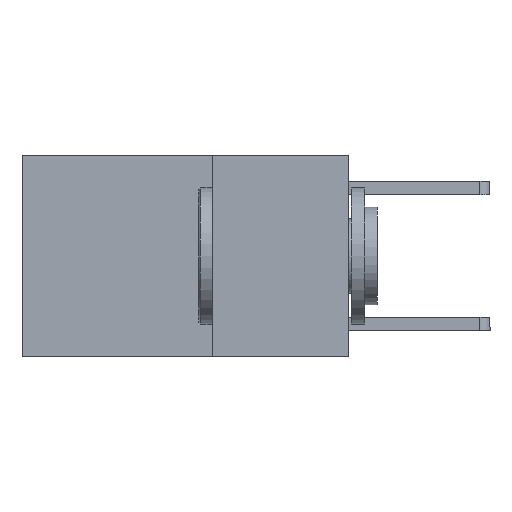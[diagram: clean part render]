
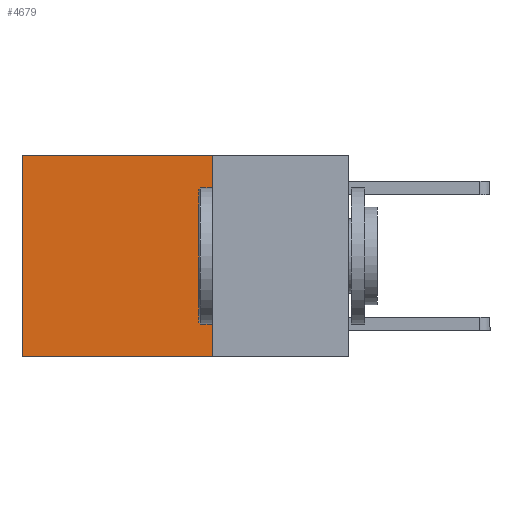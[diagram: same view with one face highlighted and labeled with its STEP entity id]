
A CAD part, left-side view. The second image highlights one B-rep face of the part: STEP entity #4679.
In plain terms, the highlighted planar face has unit normal (-1, 0, 0).
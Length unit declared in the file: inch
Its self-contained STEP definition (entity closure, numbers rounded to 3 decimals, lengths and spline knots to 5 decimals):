
#667 = LINE ( 'NONE', #8625, #9826 ) ;
#1296 = VECTOR ( 'NONE', #3431, 39.37008 ) ;
#1377 = VECTOR ( 'NONE', #4967, 39.37008 ) ;
#1406 = PLANE ( 'NONE',  #5286 ) ;
#1870 = VERTEX_POINT ( 'NONE', #2147 ) ;
#2147 = CARTESIAN_POINT ( 'NONE',  ( 0.2625, 0.25, 0. ) ) ;
#2241 = VERTEX_POINT ( 'NONE', #6012 ) ;
#2264 = DIRECTION ( 'NONE',  ( 0., 0., -1. ) ) ;
#3265 = VECTOR ( 'NONE', #11081, 39.37008 ) ;
#3323 = EDGE_LOOP ( 'NONE', ( #4667, #4480, #4279, #4560 ) ) ;
#3431 = DIRECTION ( 'NONE',  ( 0., 1., 0. ) ) ;
#3509 = EDGE_CURVE ( 'NONE', #1870, #2241, #10139, .T. ) ;
#3589 = CARTESIAN_POINT ( 'NONE',  ( 0.2625, 0.25, 0. ) ) ;
#3595 = VERTEX_POINT ( 'NONE', #7606 ) ;
#4021 = CARTESIAN_POINT ( 'NONE',  ( 0.2625, 0.25, 0. ) ) ;
#4279 = ORIENTED_EDGE ( 'NONE', *, *, #10190, .F. ) ;
#4480 = ORIENTED_EDGE ( 'NONE', *, *, #7605, .F. ) ;
#4560 = ORIENTED_EDGE ( 'NONE', *, *, #3509, .T. ) ;
#4667 = ORIENTED_EDGE ( 'NONE', *, *, #5429, .T. ) ;
#4679 = ADVANCED_FACE ( 'NONE', ( #8396 ), #1406, .F. ) ;
#4967 = DIRECTION ( 'NONE',  ( 0., 0., -1. ) ) ;
#5286 = AXIS2_PLACEMENT_3D ( 'NONE', #4021, #7714, #2264 ) ;
#5429 = EDGE_CURVE ( 'NONE', #2241, #11097, #8243, .T. ) ;
#6012 = CARTESIAN_POINT ( 'NONE',  ( 0.2625, 0.6, 0. ) ) ;
#6038 = DIRECTION ( 'NONE',  ( 0., 0., -1. ) ) ;
#7605 = EDGE_CURVE ( 'NONE', #3595, #11097, #10623, .T. ) ;
#7606 = CARTESIAN_POINT ( 'NONE',  ( 0.2625, 0.25, -0.37 ) ) ;
#7714 = DIRECTION ( 'NONE',  ( 1., 0., 0. ) ) ;
#7886 = CARTESIAN_POINT ( 'NONE',  ( 0.2625, 0.6, -0.37 ) ) ;
#8243 = LINE ( 'NONE', #10225, #1377 ) ;
#8396 = FACE_OUTER_BOUND ( 'NONE', #3323, .T. ) ;
#8625 = CARTESIAN_POINT ( 'NONE',  ( 0.2625, 0.25, 0. ) ) ;
#8665 = CARTESIAN_POINT ( 'NONE',  ( 0.2625, 0.25, -0.37 ) ) ;
#9826 = VECTOR ( 'NONE', #6038, 39.37008 ) ;
#10139 = LINE ( 'NONE', #3589, #1296 ) ;
#10190 = EDGE_CURVE ( 'NONE', #1870, #3595, #667, .T. ) ;
#10225 = CARTESIAN_POINT ( 'NONE',  ( 0.2625, 0.6, 0. ) ) ;
#10623 = LINE ( 'NONE', #8665, #3265 ) ;
#11081 = DIRECTION ( 'NONE',  ( 0., 1., 0. ) ) ;
#11097 = VERTEX_POINT ( 'NONE', #7886 ) ;
